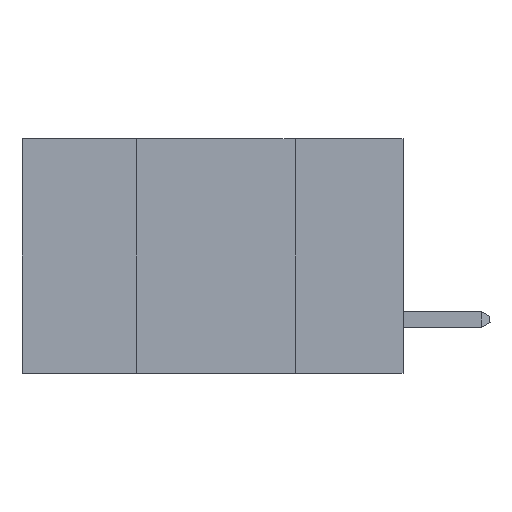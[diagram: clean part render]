
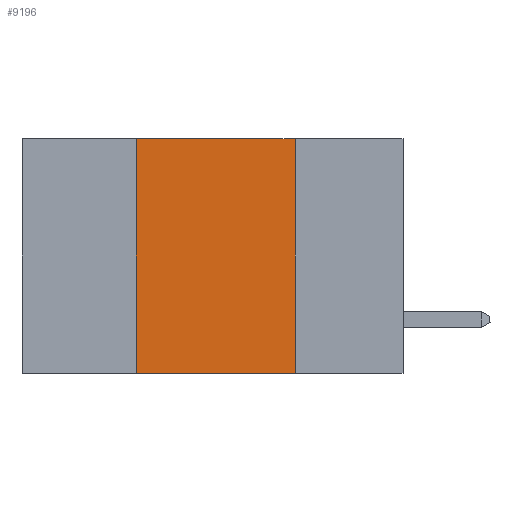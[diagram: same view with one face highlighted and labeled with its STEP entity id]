
A CAD part, left-side view. The second image highlights one B-rep face of the part: STEP entity #9196.
In plain terms, the highlighted planar face has unit normal (-1, 0, 0).
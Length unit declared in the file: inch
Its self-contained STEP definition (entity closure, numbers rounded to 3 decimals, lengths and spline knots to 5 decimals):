
#1107 = CARTESIAN_POINT ( 'NONE',  ( 0., 0.42, 0. ) ) ;
#2599 = CARTESIAN_POINT ( 'NONE',  ( 0., 0.6, 0. ) ) ;
#4780 = LINE ( 'NONE', #25865, #22572 ) ;
#5058 = DIRECTION ( 'NONE',  ( 1., 0., 0. ) ) ;
#5423 = DIRECTION ( 'NONE',  ( 0., 0., -1. ) ) ;
#6018 = VECTOR ( 'NONE', #11359, 39.37008 ) ;
#6861 = DIRECTION ( 'NONE',  ( 0., -1., 0. ) ) ;
#9196 = ADVANCED_FACE ( 'NONE', ( #21217 ), #15263, .F. ) ;
#9967 = EDGE_CURVE ( 'NONE', #12645, #13442, #10527, .T. ) ;
#10527 = LINE ( 'NONE', #18081, #22462 ) ;
#11359 = DIRECTION ( 'NONE',  ( 0., 0., 1. ) ) ;
#11752 = CARTESIAN_POINT ( 'NONE',  ( 0., 0.42, 0. ) ) ;
#12608 = EDGE_LOOP ( 'NONE', ( #15443, #24027, #24972, #12702 ) ) ;
#12645 = VERTEX_POINT ( 'NONE', #21224 ) ;
#12702 = ORIENTED_EDGE ( 'NONE', *, *, #9967, .T. ) ;
#13119 = AXIS2_PLACEMENT_3D ( 'NONE', #2599, #5058, #5423 ) ;
#13442 = VERTEX_POINT ( 'NONE', #25964 ) ;
#13514 = CARTESIAN_POINT ( 'NONE',  ( 0., 0.6, 0. ) ) ;
#15263 = PLANE ( 'NONE',  #13119 ) ;
#15443 = ORIENTED_EDGE ( 'NONE', *, *, #18288, .F. ) ;
#16188 = EDGE_CURVE ( 'NONE', #12645, #22658, #25717, .T. ) ;
#17683 = CARTESIAN_POINT ( 'NONE',  ( 0., 0.17, 0. ) ) ;
#18081 = CARTESIAN_POINT ( 'NONE',  ( 0., 0.6, -0.37 ) ) ;
#18288 = EDGE_CURVE ( 'NONE', #26485, #13442, #4780, .T. ) ;
#21217 = FACE_OUTER_BOUND ( 'NONE', #12608, .T. ) ;
#21224 = CARTESIAN_POINT ( 'NONE',  ( 0., 0.42, -0.37 ) ) ;
#21857 = DIRECTION ( 'NONE',  ( 0., -1., 0. ) ) ;
#21985 = DIRECTION ( 'NONE',  ( 0., 0., -1. ) ) ;
#22462 = VECTOR ( 'NONE', #6861, 39.37008 ) ;
#22572 = VECTOR ( 'NONE', #21985, 39.37008 ) ;
#22658 = VERTEX_POINT ( 'NONE', #11752 ) ;
#23535 = LINE ( 'NONE', #13514, #24815 ) ;
#24027 = ORIENTED_EDGE ( 'NONE', *, *, #26474, .F. ) ;
#24815 = VECTOR ( 'NONE', #21857, 39.37008 ) ;
#24972 = ORIENTED_EDGE ( 'NONE', *, *, #16188, .F. ) ;
#25717 = LINE ( 'NONE', #1107, #6018 ) ;
#25865 = CARTESIAN_POINT ( 'NONE',  ( 0., 0.17, 0. ) ) ;
#25964 = CARTESIAN_POINT ( 'NONE',  ( 0., 0.17, -0.37 ) ) ;
#26474 = EDGE_CURVE ( 'NONE', #22658, #26485, #23535, .T. ) ;
#26485 = VERTEX_POINT ( 'NONE', #17683 ) ;
